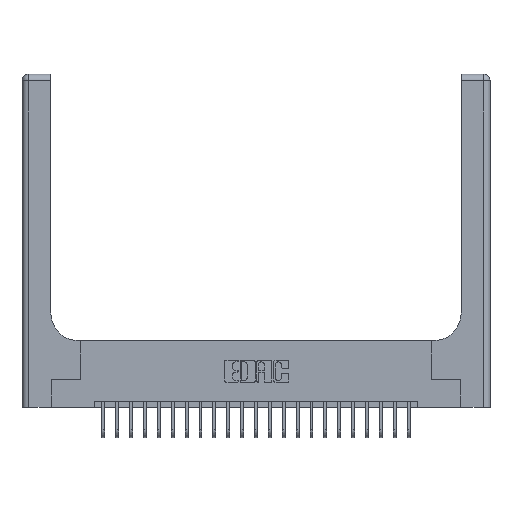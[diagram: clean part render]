
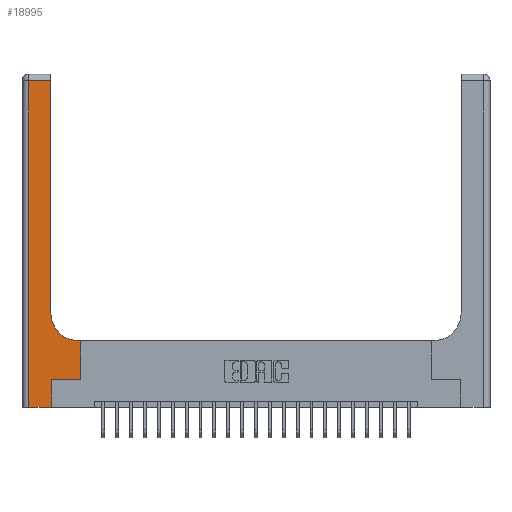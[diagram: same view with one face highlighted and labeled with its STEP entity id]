
A CAD part, top view. The second image highlights one B-rep face of the part: STEP entity #18995.
In plain terms, the highlighted planar face has unit normal (0, 0, 1).
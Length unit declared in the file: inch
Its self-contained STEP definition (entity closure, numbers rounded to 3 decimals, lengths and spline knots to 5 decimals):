
#406 = VECTOR ( 'NONE', #4023, 39.37008 ) ;
#429 = DIRECTION ( 'NONE',  ( 0., 0., -1. ) ) ;
#536 = CARTESIAN_POINT ( 'NONE',  ( 0.51, 0.85, 0.37 ) ) ;
#690 = VERTEX_POINT ( 'NONE', #8095 ) ;
#1207 = LINE ( 'NONE', #18652, #9786 ) ;
#1650 = LINE ( 'NONE', #12144, #2869 ) ;
#1736 = ORIENTED_EDGE ( 'NONE', *, *, #19201, .T. ) ;
#2369 = DIRECTION ( 'NONE',  ( 0., 1., 0. ) ) ;
#2471 = CARTESIAN_POINT ( 'NONE',  ( 0.26, 0.85, 0.37 ) ) ;
#2869 = VECTOR ( 'NONE', #3247, 39.37008 ) ;
#2908 = ORIENTED_EDGE ( 'NONE', *, *, #5194, .T. ) ;
#3019 = ORIENTED_EDGE ( 'NONE', *, *, #12742, .T. ) ;
#3247 = DIRECTION ( 'NONE',  ( -1., 0., 0. ) ) ;
#3300 = VERTEX_POINT ( 'NONE', #12943 ) ;
#3540 = ORIENTED_EDGE ( 'NONE', *, *, #7207, .T. ) ;
#3808 = EDGE_CURVE ( 'NONE', #3300, #21342, #13480, .T. ) ;
#4023 = DIRECTION ( 'NONE',  ( 0., 1., 0. ) ) ;
#4135 = ORIENTED_EDGE ( 'NONE', *, *, #22503, .T. ) ;
#4747 = DIRECTION ( 'NONE',  ( 1., 0., 0. ) ) ;
#5049 = DIRECTION ( 'NONE',  ( 0., 1., 0. ) ) ;
#5194 = EDGE_CURVE ( 'NONE', #12675, #21609, #21420, .T. ) ;
#5290 = LINE ( 'NONE', #17500, #406 ) ;
#5814 = VECTOR ( 'NONE', #7711, 39.37008 ) ;
#5942 = AXIS2_PLACEMENT_3D ( 'NONE', #536, #9198, #13083 ) ;
#6025 = CARTESIAN_POINT ( 'NONE',  ( 0.265, 0.25, 0.37 ) ) ;
#6029 = CARTESIAN_POINT ( 'NONE',  ( 0.26, 2.94, 0.37 ) ) ;
#6186 = VERTEX_POINT ( 'NONE', #17363 ) ;
#6693 = EDGE_CURVE ( 'NONE', #6186, #690, #11249, .T. ) ;
#6707 = ORIENTED_EDGE ( 'NONE', *, *, #6693, .T. ) ;
#6946 = DIRECTION ( 'NONE',  ( -1., 0., 0. ) ) ;
#7162 = CARTESIAN_POINT ( 'NONE',  ( 0.265, 0., 0.37 ) ) ;
#7207 = EDGE_CURVE ( 'NONE', #19915, #14125, #8362, .T. ) ;
#7432 = CARTESIAN_POINT ( 'NONE',  ( 0.528, 0.25, 0.37 ) ) ;
#7448 = VECTOR ( 'NONE', #18001, 39.37008 ) ;
#7711 = DIRECTION ( 'NONE',  ( 0., -1., 0. ) ) ;
#7811 = CARTESIAN_POINT ( 'NONE',  ( 0.51, 0.6, 0.37 ) ) ;
#8076 = EDGE_CURVE ( 'NONE', #16907, #3300, #5290, .T. ) ;
#8095 = CARTESIAN_POINT ( 'NONE',  ( 0.06, 0., 0.37 ) ) ;
#8271 = VECTOR ( 'NONE', #18597, 39.37008 ) ;
#8362 = LINE ( 'NONE', #18615, #18576 ) ;
#9198 = DIRECTION ( 'NONE',  ( 0., 0., -1. ) ) ;
#9786 = VECTOR ( 'NONE', #4747, 39.37008 ) ;
#10829 = AXIS2_PLACEMENT_3D ( 'NONE', #15727, #429, #6946 ) ;
#11249 = LINE ( 'NONE', #18198, #5814 ) ;
#11260 = ORIENTED_EDGE ( 'NONE', *, *, #12470, .T. ) ;
#12144 = CARTESIAN_POINT ( 'NONE',  ( 0., 2.94, 0.37 ) ) ;
#12470 = EDGE_CURVE ( 'NONE', #21609, #16907, #21767, .T. ) ;
#12675 = VERTEX_POINT ( 'NONE', #7162 ) ;
#12742 = EDGE_CURVE ( 'NONE', #21342, #19915, #15792, .T. ) ;
#12943 = CARTESIAN_POINT ( 'NONE',  ( 0.528, 0.6, 0.37 ) ) ;
#13083 = DIRECTION ( 'NONE',  ( 1., 0., 0. ) ) ;
#13112 = VECTOR ( 'NONE', #2369, 39.37008 ) ;
#13480 = LINE ( 'NONE', #16895, #8271 ) ;
#14125 = VERTEX_POINT ( 'NONE', #6029 ) ;
#15727 = CARTESIAN_POINT ( 'NONE',  ( 0., 3., 0.37 ) ) ;
#15792 = CIRCLE ( 'NONE', #5942, 0.25 ) ;
#16052 = PLANE ( 'NONE',  #10829 ) ;
#16895 = CARTESIAN_POINT ( 'NONE',  ( 0.26, 0.6, 0.37 ) ) ;
#16907 = VERTEX_POINT ( 'NONE', #7432 ) ;
#17363 = CARTESIAN_POINT ( 'NONE',  ( 0.06, 2.94, 0.37 ) ) ;
#17500 = CARTESIAN_POINT ( 'NONE',  ( 0.528, 0.25, 0.37 ) ) ;
#17845 = ORIENTED_EDGE ( 'NONE', *, *, #3808, .T. ) ;
#18001 = DIRECTION ( 'NONE',  ( 1., 0., 0. ) ) ;
#18198 = CARTESIAN_POINT ( 'NONE',  ( 0.06, 3., 0.37 ) ) ;
#18576 = VECTOR ( 'NONE', #5049, 39.37008 ) ;
#18597 = DIRECTION ( 'NONE',  ( -1., 0., 0. ) ) ;
#18615 = CARTESIAN_POINT ( 'NONE',  ( 0.26, 3., 0.37 ) ) ;
#18652 = CARTESIAN_POINT ( 'NONE',  ( 0., 0., 0.37 ) ) ;
#18995 = ADVANCED_FACE ( 'NONE', ( #20857 ), #16052, .F. ) ;
#19201 = EDGE_CURVE ( 'NONE', #690, #12675, #1207, .T. ) ;
#19398 = EDGE_LOOP ( 'NONE', ( #3540, #4135, #6707, #1736, #2908, #11260, #20663, #17845, #3019 ) ) ;
#19703 = CARTESIAN_POINT ( 'NONE',  ( 0.265, 0., 0.37 ) ) ;
#19915 = VERTEX_POINT ( 'NONE', #2471 ) ;
#20663 = ORIENTED_EDGE ( 'NONE', *, *, #8076, .T. ) ;
#20857 = FACE_OUTER_BOUND ( 'NONE', #19398, .T. ) ;
#21342 = VERTEX_POINT ( 'NONE', #7811 ) ;
#21420 = LINE ( 'NONE', #19703, #13112 ) ;
#21609 = VERTEX_POINT ( 'NONE', #21693 ) ;
#21693 = CARTESIAN_POINT ( 'NONE',  ( 0.265, 0.25, 0.37 ) ) ;
#21767 = LINE ( 'NONE', #6025, #7448 ) ;
#22503 = EDGE_CURVE ( 'NONE', #14125, #6186, #1650, .T. ) ;
